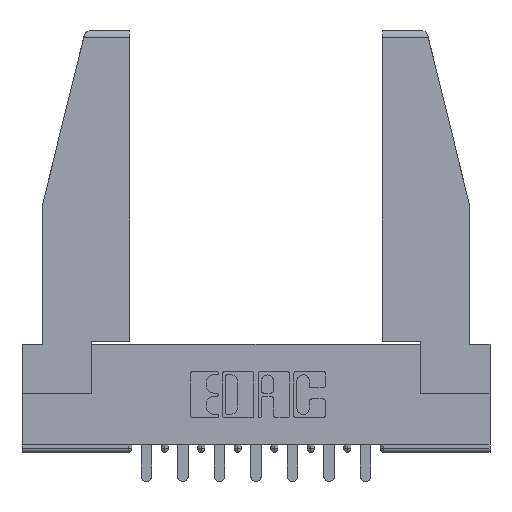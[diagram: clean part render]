
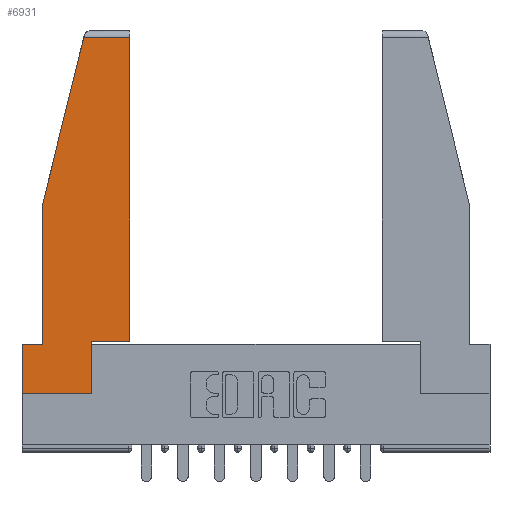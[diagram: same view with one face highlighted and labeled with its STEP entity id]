
A CAD part, top view. The second image highlights one B-rep face of the part: STEP entity #6931.
In plain terms, the highlighted planar face has unit normal (0, 0, 1).
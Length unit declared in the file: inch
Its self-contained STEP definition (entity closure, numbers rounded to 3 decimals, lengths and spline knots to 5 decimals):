
#65 = CARTESIAN_POINT ( 'NONE',  ( 0.086, 0.8, 0. ) ) ;
#109 = CARTESIAN_POINT ( 'NONE',  ( 0.461, 0.223, 0. ) ) ;
#159 = DIRECTION ( 'NONE',  ( 0., -1., 0. ) ) ;
#345 = LINE ( 'NONE', #8582, #11659 ) ;
#675 = DIRECTION ( 'NONE',  ( 1., 0., 0. ) ) ;
#698 = VECTOR ( 'NONE', #3388, 39.37008 ) ;
#726 = ORIENTED_EDGE ( 'NONE', *, *, #7615, .T. ) ;
#884 = VERTEX_POINT ( 'NONE', #12615 ) ;
#943 = VECTOR ( 'NONE', #2204, 39.37008 ) ;
#1013 = EDGE_CURVE ( 'NONE', #884, #9205, #11015, .T. ) ;
#1578 = DIRECTION ( 'NONE',  ( 1., 0., 0. ) ) ;
#2190 = DIRECTION ( 'NONE',  ( -0.239, -0.971, 0. ) ) ;
#2204 = DIRECTION ( 'NONE',  ( -1., 0., 0. ) ) ;
#2409 = EDGE_CURVE ( 'NONE', #5448, #3474, #3430, .T. ) ;
#2419 = EDGE_CURVE ( 'NONE', #6379, #10212, #345, .T. ) ;
#2567 = LINE ( 'NONE', #5445, #5523 ) ;
#2680 = CARTESIAN_POINT ( 'NONE',  ( 0.297, 0., 0. ) ) ;
#3325 = CARTESIAN_POINT ( 'NONE',  ( 0., 1.52, 0. ) ) ;
#3388 = DIRECTION ( 'NONE',  ( 0., -1., 0. ) ) ;
#3430 = LINE ( 'NONE', #109, #9751 ) ;
#3474 = VERTEX_POINT ( 'NONE', #13949 ) ;
#3847 = DIRECTION ( 'NONE',  ( 0., 1., 0. ) ) ;
#3850 = EDGE_LOOP ( 'NONE', ( #11895, #8373, #8904, #726, #10919, #11491, #9611, #9994, #8050 ) ) ;
#4100 = PLANE ( 'NONE',  #10582 ) ;
#4743 = VECTOR ( 'NONE', #3847, 39.37008 ) ;
#4813 = EDGE_CURVE ( 'NONE', #3474, #14114, #8027, .T. ) ;
#4843 = VECTOR ( 'NONE', #159, 39.37008 ) ;
#5256 = CARTESIAN_POINT ( 'NONE',  ( 0., 0.21, 0. ) ) ;
#5303 = DIRECTION ( 'NONE',  ( -1., 0., 0. ) ) ;
#5445 = CARTESIAN_POINT ( 'NONE',  ( 0.271, 1.55, 0. ) ) ;
#5448 = VERTEX_POINT ( 'NONE', #7143 ) ;
#5523 = VECTOR ( 'NONE', #2190, 39.37008 ) ;
#5695 = LINE ( 'NONE', #10218, #12661 ) ;
#5953 = DIRECTION ( 'NONE',  ( 0., 1., 0. ) ) ;
#6379 = VERTEX_POINT ( 'NONE', #10072 ) ;
#6931 = ADVANCED_FACE ( 'NONE', ( #9292 ), #4100, .T. ) ;
#6941 = VECTOR ( 'NONE', #5303, 39.37008 ) ;
#7143 = CARTESIAN_POINT ( 'NONE',  ( 0.461, 0.223, 0. ) ) ;
#7288 = DIRECTION ( 'NONE',  ( 0., 0., 1. ) ) ;
#7615 = EDGE_CURVE ( 'NONE', #9539, #884, #8933, .T. ) ;
#7656 = LINE ( 'NONE', #2680, #4743 ) ;
#7738 = CARTESIAN_POINT ( 'NONE',  ( 0., 0.21, 0. ) ) ;
#7876 = VERTEX_POINT ( 'NONE', #13561 ) ;
#8027 = LINE ( 'NONE', #3325, #943 ) ;
#8050 = ORIENTED_EDGE ( 'NONE', *, *, #10835, .T. ) ;
#8373 = ORIENTED_EDGE ( 'NONE', *, *, #4813, .T. ) ;
#8582 = CARTESIAN_POINT ( 'NONE',  ( 0., 0., 0. ) ) ;
#8644 = EDGE_CURVE ( 'NONE', #9205, #6379, #14192, .T. ) ;
#8904 = ORIENTED_EDGE ( 'NONE', *, *, #9199, .T. ) ;
#8933 = LINE ( 'NONE', #65, #698 ) ;
#9199 = EDGE_CURVE ( 'NONE', #14114, #9539, #2567, .T. ) ;
#9205 = VERTEX_POINT ( 'NONE', #7738 ) ;
#9292 = FACE_OUTER_BOUND ( 'NONE', #3850, .T. ) ;
#9357 = CARTESIAN_POINT ( 'NONE',  ( 0.297, 0., 0. ) ) ;
#9539 = VERTEX_POINT ( 'NONE', #12717 ) ;
#9611 = ORIENTED_EDGE ( 'NONE', *, *, #2419, .T. ) ;
#9751 = VECTOR ( 'NONE', #5953, 39.37008 ) ;
#9994 = ORIENTED_EDGE ( 'NONE', *, *, #13370, .T. ) ;
#10072 = CARTESIAN_POINT ( 'NONE',  ( 0., 0., 0. ) ) ;
#10172 = CARTESIAN_POINT ( 'NONE',  ( 0.2636, 1.52, 0. ) ) ;
#10212 = VERTEX_POINT ( 'NONE', #9357 ) ;
#10218 = CARTESIAN_POINT ( 'NONE',  ( 0.297, 0.223, 0. ) ) ;
#10582 = AXIS2_PLACEMENT_3D ( 'NONE', #12699, #7288, #675 ) ;
#10835 = EDGE_CURVE ( 'NONE', #7876, #5448, #5695, .T. ) ;
#10919 = ORIENTED_EDGE ( 'NONE', *, *, #1013, .T. ) ;
#11015 = LINE ( 'NONE', #5256, #6941 ) ;
#11421 = DIRECTION ( 'NONE',  ( 1., 0., 0. ) ) ;
#11491 = ORIENTED_EDGE ( 'NONE', *, *, #8644, .T. ) ;
#11659 = VECTOR ( 'NONE', #11421, 39.37008 ) ;
#11895 = ORIENTED_EDGE ( 'NONE', *, *, #2409, .T. ) ;
#12138 = CARTESIAN_POINT ( 'NONE',  ( 0., 0.21, 0. ) ) ;
#12615 = CARTESIAN_POINT ( 'NONE',  ( 0.086, 0.21, 0. ) ) ;
#12661 = VECTOR ( 'NONE', #1578, 39.37008 ) ;
#12699 = CARTESIAN_POINT ( 'NONE',  ( 0., 0., 0. ) ) ;
#12717 = CARTESIAN_POINT ( 'NONE',  ( 0.086, 0.8, 0. ) ) ;
#13370 = EDGE_CURVE ( 'NONE', #10212, #7876, #7656, .T. ) ;
#13561 = CARTESIAN_POINT ( 'NONE',  ( 0.297, 0.223, 0. ) ) ;
#13949 = CARTESIAN_POINT ( 'NONE',  ( 0.461, 1.52, 0. ) ) ;
#14114 = VERTEX_POINT ( 'NONE', #10172 ) ;
#14192 = LINE ( 'NONE', #12138, #4843 ) ;
